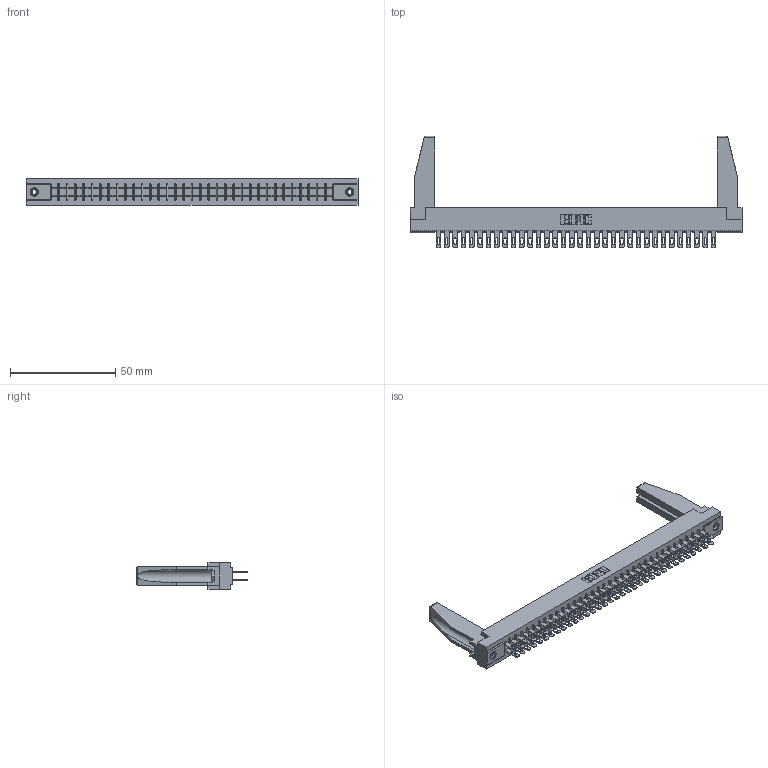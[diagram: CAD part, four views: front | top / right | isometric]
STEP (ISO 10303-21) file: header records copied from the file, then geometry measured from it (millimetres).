
FILE_DESCRIPTION (( 'STEP AP203' ), '1' );
FILE_NAME ('355-068-500-578.STEP', '2019-09-12T16:48:59', ( '' ), ( '' ), 'SwSTEP 2.0', 'SolidWorks 2016', '' );
FILE_SCHEMA (( 'CONFIG_CONTROL_DESIGN' ));
Length unit declared in the file: inch
Products named in the file (5): 345-250-001_345-250-001-102; 307-220-078; 305 Part_.156 Dia; 355-068-500-578; 305-290-001_500
Assembly tree (73 placements, depth 2):
  355-068-500-578
    305 Part_.156 Dia
    305-290-001_500  x68
    345-250-001_345-250-001-102  x2
    307-220-078  x2
Bounding box: 157.73 x 52.88 x 12.7 mm (x, y, z)
Volume: 20140.2 mm3; surface area: 26271.5 mm2
Topology: 73 solids, 73 shells, 3646 faces, 10404 edges, 6744 vertices
Faces by surface type: plane 2056, cylinder 1438, sphere 136, cone 12, torus 4
Entity records: 40248 total; most frequent: CARTESIAN_POINT 6666, ORIENTED_EDGE 6574, DIRECTION 6415, EDGE_CURVE 3287, VECTOR 2645, LINE 2645, VERTEX_POINT 2094, AXIS2_PLACEMENT_3D 1885
